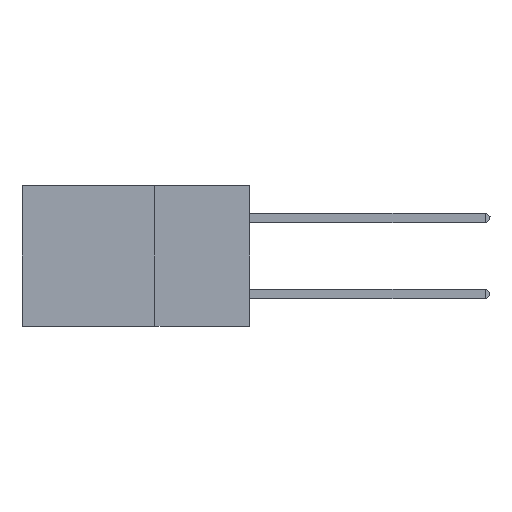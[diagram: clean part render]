
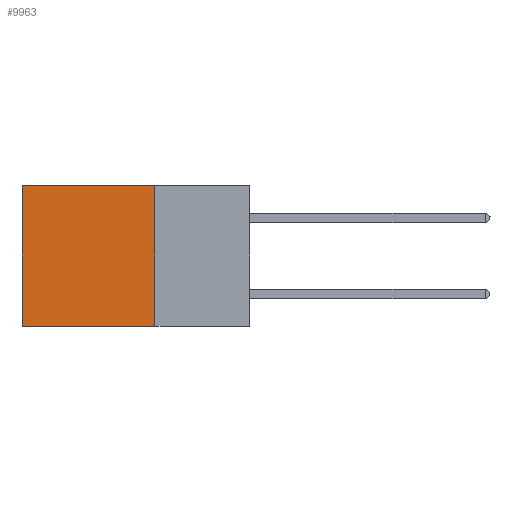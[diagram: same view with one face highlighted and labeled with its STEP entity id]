
A CAD part, left-side view. The second image highlights one B-rep face of the part: STEP entity #9963.
In plain terms, the highlighted planar face has unit normal (-1, 0, 0).
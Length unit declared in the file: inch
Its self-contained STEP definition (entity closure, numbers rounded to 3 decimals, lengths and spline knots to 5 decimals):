
#317 = VERTEX_POINT ( 'NONE', #1380 ) ;
#1252 = EDGE_CURVE ( 'NONE', #6916, #317, #23358, .T. ) ;
#1380 = CARTESIAN_POINT ( 'NONE',  ( 0.2875, 0.25, -0.37 ) ) ;
#1740 = DIRECTION ( 'NONE',  ( 0., 1., 0. ) ) ;
#2130 = CARTESIAN_POINT ( 'NONE',  ( 0.2875, 0.6, 0. ) ) ;
#2979 = FACE_OUTER_BOUND ( 'NONE', #8567, .T. ) ;
#3454 = CARTESIAN_POINT ( 'NONE',  ( 0.2875, 0.25, 0. ) ) ;
#4255 = CARTESIAN_POINT ( 'NONE',  ( 0.2875, 0.6, 0. ) ) ;
#4624 = DIRECTION ( 'NONE',  ( 1., 0., 0. ) ) ;
#5687 = LINE ( 'NONE', #7714, #18187 ) ;
#6041 = CARTESIAN_POINT ( 'NONE',  ( 0.2875, 0.25, 0. ) ) ;
#6797 = VECTOR ( 'NONE', #15537, 39.37008 ) ;
#6916 = VERTEX_POINT ( 'NONE', #3454 ) ;
#7714 = CARTESIAN_POINT ( 'NONE',  ( 0.2875, 0.25, 0. ) ) ;
#8433 = AXIS2_PLACEMENT_3D ( 'NONE', #21807, #4624, #12326 ) ;
#8567 = EDGE_LOOP ( 'NONE', ( #21403, #11384, #22299, #21539 ) ) ;
#9205 = CARTESIAN_POINT ( 'NONE',  ( 0.2875, 0.25, -0.37 ) ) ;
#9325 = LINE ( 'NONE', #9205, #23538 ) ;
#9426 = EDGE_CURVE ( 'NONE', #20239, #12990, #11724, .T. ) ;
#9963 = ADVANCED_FACE ( 'NONE', ( #2979 ), #10305, .F. ) ;
#10305 = PLANE ( 'NONE',  #8433 ) ;
#11384 = ORIENTED_EDGE ( 'NONE', *, *, #20142, .F. ) ;
#11724 = LINE ( 'NONE', #2130, #6797 ) ;
#12326 = DIRECTION ( 'NONE',  ( 0., 0., -1. ) ) ;
#12643 = VECTOR ( 'NONE', #16163, 39.37008 ) ;
#12990 = VERTEX_POINT ( 'NONE', #15518 ) ;
#15429 = DIRECTION ( 'NONE',  ( 0., 1., 0. ) ) ;
#15518 = CARTESIAN_POINT ( 'NONE',  ( 0.2875, 0.6, -0.37 ) ) ;
#15537 = DIRECTION ( 'NONE',  ( 0., 0., -1. ) ) ;
#16163 = DIRECTION ( 'NONE',  ( 0., 0., -1. ) ) ;
#17077 = EDGE_CURVE ( 'NONE', #6916, #20239, #5687, .T. ) ;
#18187 = VECTOR ( 'NONE', #15429, 39.37008 ) ;
#20142 = EDGE_CURVE ( 'NONE', #317, #12990, #9325, .T. ) ;
#20239 = VERTEX_POINT ( 'NONE', #4255 ) ;
#21403 = ORIENTED_EDGE ( 'NONE', *, *, #9426, .T. ) ;
#21539 = ORIENTED_EDGE ( 'NONE', *, *, #17077, .T. ) ;
#21807 = CARTESIAN_POINT ( 'NONE',  ( 0.2875, 0.25, 0. ) ) ;
#22299 = ORIENTED_EDGE ( 'NONE', *, *, #1252, .F. ) ;
#23358 = LINE ( 'NONE', #6041, #12643 ) ;
#23538 = VECTOR ( 'NONE', #1740, 39.37008 ) ;
